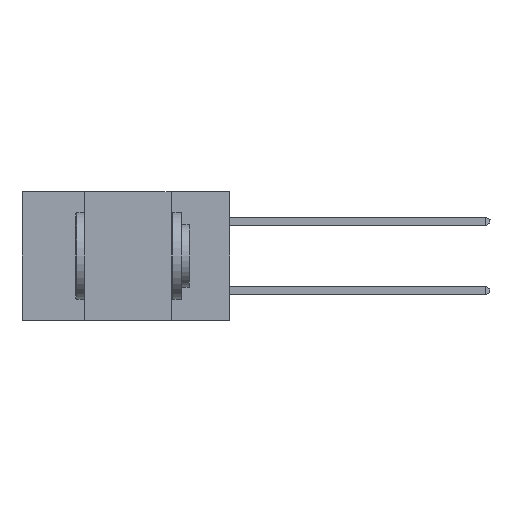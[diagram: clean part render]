
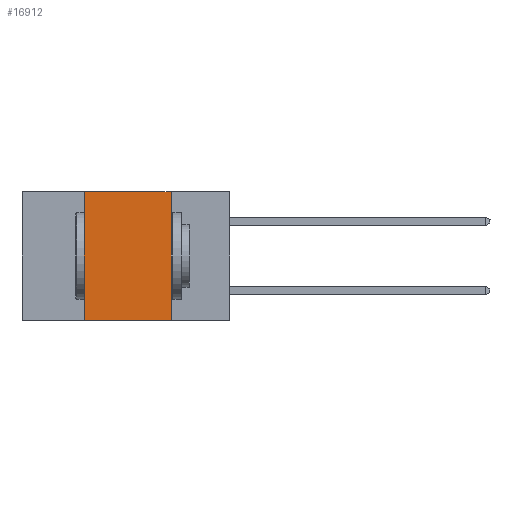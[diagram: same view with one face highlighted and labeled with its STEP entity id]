
A CAD part, left-side view. The second image highlights one B-rep face of the part: STEP entity #16912.
In plain terms, the highlighted planar face has unit normal (-1, 0, 0).
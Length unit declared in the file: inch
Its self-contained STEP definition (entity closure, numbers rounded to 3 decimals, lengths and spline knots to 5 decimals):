
#1193 = CARTESIAN_POINT ( 'NONE',  ( 0., 0.17, 0. ) ) ;
#1614 = CARTESIAN_POINT ( 'NONE',  ( 0., 0.6, 0. ) ) ;
#2126 = AXIS2_PLACEMENT_3D ( 'NONE', #7253, #16707, #9967 ) ;
#2160 = EDGE_CURVE ( 'NONE', #3398, #3842, #17176, .T. ) ;
#2547 = CARTESIAN_POINT ( 'NONE',  ( 0., 0.42, 0. ) ) ;
#2796 = DIRECTION ( 'NONE',  ( 0., -1., 0. ) ) ;
#3398 = VERTEX_POINT ( 'NONE', #1193 ) ;
#3736 = LINE ( 'NONE', #4248, #6236 ) ;
#3769 = EDGE_CURVE ( 'NONE', #12911, #3842, #12140, .T. ) ;
#3842 = VERTEX_POINT ( 'NONE', #10199 ) ;
#4174 = VERTEX_POINT ( 'NONE', #2547 ) ;
#4248 = CARTESIAN_POINT ( 'NONE',  ( 0., 0.42, 0. ) ) ;
#4271 = ORIENTED_EDGE ( 'NONE', *, *, #2160, .F. ) ;
#5282 = DIRECTION ( 'NONE',  ( 0., 0., -1. ) ) ;
#6236 = VECTOR ( 'NONE', #16289, 39.37008 ) ;
#7227 = VECTOR ( 'NONE', #5282, 39.37008 ) ;
#7253 = CARTESIAN_POINT ( 'NONE',  ( 0., 0.6, 0. ) ) ;
#8862 = EDGE_CURVE ( 'NONE', #12911, #4174, #3736, .T. ) ;
#9169 = CARTESIAN_POINT ( 'NONE',  ( 0., 0.42, -0.37 ) ) ;
#9210 = VECTOR ( 'NONE', #13553, 39.37008 ) ;
#9362 = ORIENTED_EDGE ( 'NONE', *, *, #15912, .F. ) ;
#9846 = PLANE ( 'NONE',  #2126 ) ;
#9967 = DIRECTION ( 'NONE',  ( 0., 0., -1. ) ) ;
#10060 = EDGE_LOOP ( 'NONE', ( #4271, #9362, #15945, #14822 ) ) ;
#10199 = CARTESIAN_POINT ( 'NONE',  ( 0., 0.17, -0.37 ) ) ;
#10267 = VECTOR ( 'NONE', #2796, 39.37008 ) ;
#12140 = LINE ( 'NONE', #15894, #10267 ) ;
#12328 = FACE_OUTER_BOUND ( 'NONE', #10060, .T. ) ;
#12713 = CARTESIAN_POINT ( 'NONE',  ( 0., 0.17, 0. ) ) ;
#12911 = VERTEX_POINT ( 'NONE', #9169 ) ;
#13553 = DIRECTION ( 'NONE',  ( 0., -1., 0. ) ) ;
#14822 = ORIENTED_EDGE ( 'NONE', *, *, #3769, .T. ) ;
#15889 = LINE ( 'NONE', #1614, #9210 ) ;
#15894 = CARTESIAN_POINT ( 'NONE',  ( 0., 0.6, -0.37 ) ) ;
#15912 = EDGE_CURVE ( 'NONE', #4174, #3398, #15889, .T. ) ;
#15945 = ORIENTED_EDGE ( 'NONE', *, *, #8862, .F. ) ;
#16289 = DIRECTION ( 'NONE',  ( 0., 0., 1. ) ) ;
#16707 = DIRECTION ( 'NONE',  ( 1., 0., 0. ) ) ;
#16912 = ADVANCED_FACE ( 'NONE', ( #12328 ), #9846, .F. ) ;
#17176 = LINE ( 'NONE', #12713, #7227 ) ;
